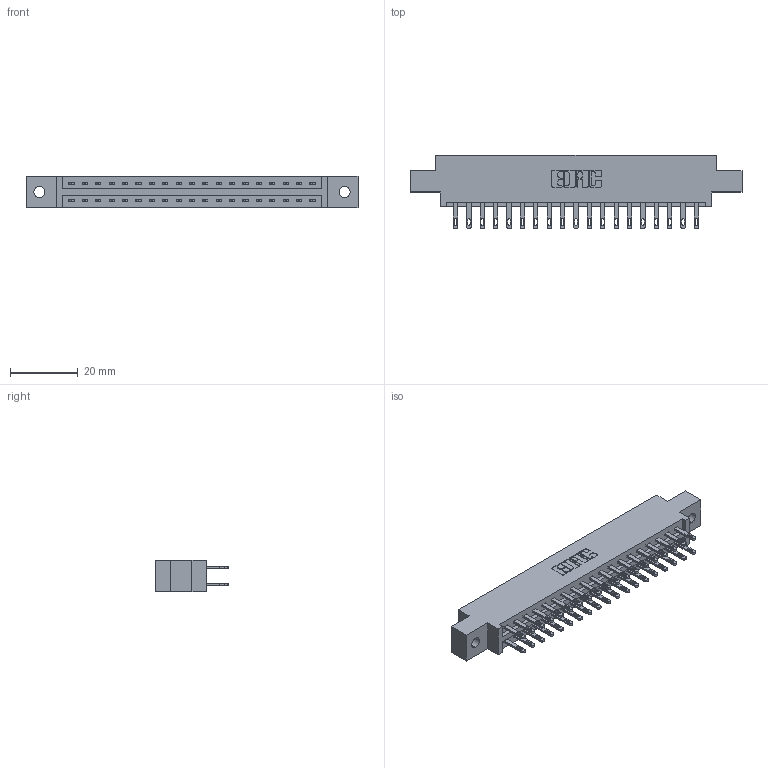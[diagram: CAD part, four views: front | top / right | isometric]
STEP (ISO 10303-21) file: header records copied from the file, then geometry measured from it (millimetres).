
FILE_DESCRIPTION (( 'STEP AP203' ), '1' );
FILE_NAME ('337-038-500-802.STEP', '2019-10-11T11:06:04', ( '' ), ( '' ), 'SwSTEP 2.0', 'SolidWorks 2016', '' );
FILE_SCHEMA (( 'CONFIG_CONTROL_DESIGN' ));
Length unit declared in the file: inch
Products named in the file (3): 337-038-500-802; 337 Part_0.170 Offset - 0.128 Dia; 345-292-001_345-293-100
Assembly tree (39 placements, depth 2):
  337-038-500-802
    337 Part_0.170 Offset - 0.128 Dia
    345-292-001_345-293-100  x38
Bounding box: 98.3 x 21.85 x 9.4 mm (x, y, z)
Volume: 10015.2 mm3; surface area: 11355.6 mm2
Topology: 39 solids, 39 shells, 2018 faces, 6137 edges, 4090 vertices
Faces by surface type: plane 1290, cylinder 728
Entity records: 17771 total; most frequent: CARTESIAN_POINT 3014, ORIENTED_EDGE 2950, DIRECTION 2607, EDGE_CURVE 1475, LINE 1343, VECTOR 1343, VERTEX_POINT 982, AXIS2_PLACEMENT_3D 632
